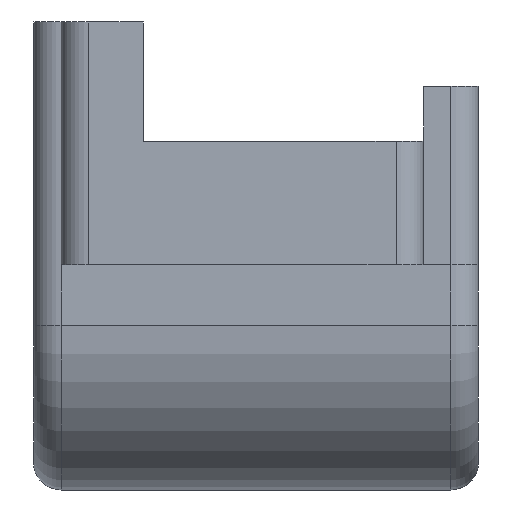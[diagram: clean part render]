
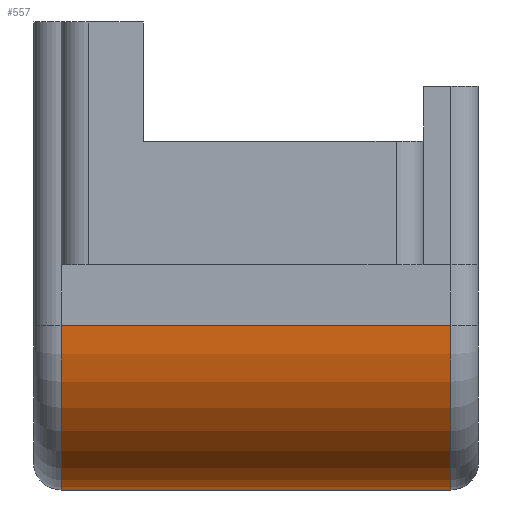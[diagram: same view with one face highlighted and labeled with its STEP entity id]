
A CAD part, left-side view. The second image highlights one B-rep face of the part: STEP entity #557.
In plain terms, the highlighted cylindrical face has radius 6 mm (diameter 12 mm), a partial arc.
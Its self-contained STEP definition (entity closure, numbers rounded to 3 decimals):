
#149 = EDGE_CURVE ( 'NONE', #1347, #369, #1127, .T. ) ;
#187 = EDGE_CURVE ( 'NONE', #708, #1680, #231, .T. ) ;
#231 = LINE ( 'NONE', #1649, #1106 ) ;
#292 = EDGE_CURVE ( 'NONE', #1347, #1680, #1465, .T. ) ;
#369 = VERTEX_POINT ( 'NONE', #1297 ) ;
#388 = DIRECTION ( 'NONE',  ( -0.707, 0., -0.707 ) ) ;
#412 = EDGE_CURVE ( 'NONE', #708, #369, #835, .T. ) ;
#436 = AXIS2_PLACEMENT_3D ( 'NONE', #1240, #694, #1500 ) ;
#455 = ORIENTED_EDGE ( 'NONE', *, *, #292, .F. ) ;
#463 = CARTESIAN_POINT ( 'NONE',  ( -93., 17.293, -33.8 ) ) ;
#470 = DIRECTION ( 'NONE',  ( 0., 1., 0. ) ) ;
#528 = ORIENTED_EDGE ( 'NONE', *, *, #412, .F. ) ;
#540 = CYLINDRICAL_SURFACE ( 'NONE', #436, 6. ) ;
#557 = ADVANCED_FACE ( 'NONE', ( #903 ), #540, .T. ) ;
#576 = CARTESIAN_POINT ( 'NONE',  ( -93., 17.043, -39.8 ) ) ;
#639 = CARTESIAN_POINT ( 'NONE',  ( -99., 17.293, -33.8 ) ) ;
#649 = AXIS2_PLACEMENT_3D ( 'NONE', #1699, #1186, #388 ) ;
#694 = DIRECTION ( 'NONE',  ( 0., 1., 0. ) ) ;
#708 = VERTEX_POINT ( 'NONE', #860 ) ;
#835 = CIRCLE ( 'NONE', #649, 6. ) ;
#842 = ORIENTED_EDGE ( 'NONE', *, *, #187, .T. ) ;
#849 = DIRECTION ( 'NONE',  ( 0., 1., 0. ) ) ;
#860 = CARTESIAN_POINT ( 'NONE',  ( -99., 3.093, -33.8 ) ) ;
#903 = FACE_OUTER_BOUND ( 'NONE', #1301, .T. ) ;
#1106 = VECTOR ( 'NONE', #849, 1000. ) ;
#1127 = LINE ( 'NONE', #576, #1507 ) ;
#1154 = ORIENTED_EDGE ( 'NONE', *, *, #149, .T. ) ;
#1186 = DIRECTION ( 'NONE',  ( 0., -1., 0. ) ) ;
#1240 = CARTESIAN_POINT ( 'NONE',  ( -93., 17.043, -33.8 ) ) ;
#1297 = CARTESIAN_POINT ( 'NONE',  ( -93., 3.093, -39.8 ) ) ;
#1301 = EDGE_LOOP ( 'NONE', ( #455, #1154, #528, #842 ) ) ;
#1305 = AXIS2_PLACEMENT_3D ( 'NONE', #463, #470, #1398 ) ;
#1347 = VERTEX_POINT ( 'NONE', #1706 ) ;
#1398 = DIRECTION ( 'NONE',  ( -0.707, 0., -0.707 ) ) ;
#1465 = CIRCLE ( 'NONE', #1305, 6. ) ;
#1500 = DIRECTION ( 'NONE',  ( -0.707, 0., -0.707 ) ) ;
#1507 = VECTOR ( 'NONE', #1661, 1000. ) ;
#1649 = CARTESIAN_POINT ( 'NONE',  ( -99., 17.043, -33.8 ) ) ;
#1661 = DIRECTION ( 'NONE',  ( 0., -1., 0. ) ) ;
#1680 = VERTEX_POINT ( 'NONE', #639 ) ;
#1699 = CARTESIAN_POINT ( 'NONE',  ( -93., 3.093, -33.8 ) ) ;
#1706 = CARTESIAN_POINT ( 'NONE',  ( -93., 17.293, -39.8 ) ) ;
